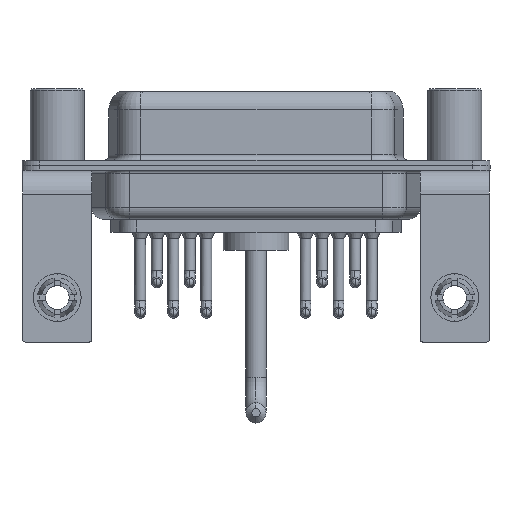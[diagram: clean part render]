
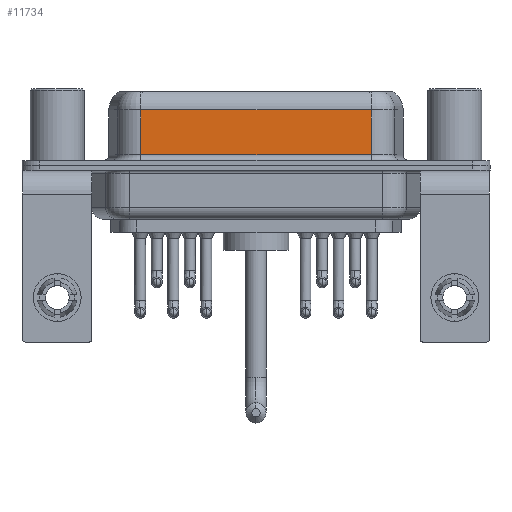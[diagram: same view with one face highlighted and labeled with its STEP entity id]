
A CAD part, front view. The second image highlights one B-rep face of the part: STEP entity #11734.
In plain terms, the highlighted planar face has unit normal (0, -1, 0).
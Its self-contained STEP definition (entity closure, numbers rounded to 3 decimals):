
#398 = DIRECTION ( 'NONE',  ( -1., 0., 0. ) ) ;
#414 = DIRECTION ( 'NONE',  ( 1., 0., 0. ) ) ;
#1727 = LINE ( 'NONE', #19371, #4014 ) ;
#2548 = VERTEX_POINT ( 'NONE', #21222 ) ;
#3657 = CARTESIAN_POINT ( 'NONE',  ( 26.287, -3.95, 6.4 ) ) ;
#3680 = DIRECTION ( 'NONE',  ( 0., 0., -1. ) ) ;
#4014 = VECTOR ( 'NONE', #3680, 1000. ) ;
#4272 = EDGE_CURVE ( 'NONE', #6927, #19515, #12548, .T. ) ;
#4335 = EDGE_CURVE ( 'NONE', #2548, #19515, #21192, .T. ) ;
#4489 = VECTOR ( 'NONE', #398, 1000. ) ;
#5898 = CARTESIAN_POINT ( 'NONE',  ( 7.013, -3.95, 4.65 ) ) ;
#6927 = VERTEX_POINT ( 'NONE', #22051 ) ;
#7411 = EDGE_LOOP ( 'NONE', ( #15290, #13321, #18387, #22272 ) ) ;
#8195 = DIRECTION ( 'NONE',  ( 0., 0., 1. ) ) ;
#8648 = VECTOR ( 'NONE', #414, 1000. ) ;
#9180 = CARTESIAN_POINT ( 'NONE',  ( 26.287, -3.95, 4.65 ) ) ;
#9944 = CARTESIAN_POINT ( 'NONE',  ( 26.287, -3.95, 6.4 ) ) ;
#10717 = DIRECTION ( 'NONE',  ( 0., 0., -1. ) ) ;
#11469 = AXIS2_PLACEMENT_3D ( 'NONE', #9944, #15365, #8195 ) ;
#11734 = ADVANCED_FACE ( 'NONE', ( #15143 ), #13510, .F. ) ;
#12199 = CARTESIAN_POINT ( 'NONE',  ( 26.287, -3.95, 0.9 ) ) ;
#12548 = LINE ( 'NONE', #12199, #8648 ) ;
#12831 = CARTESIAN_POINT ( 'NONE',  ( 26.287, -3.95, 0.9 ) ) ;
#13321 = ORIENTED_EDGE ( 'NONE', *, *, #22125, .T. ) ;
#13510 = PLANE ( 'NONE',  #11469 ) ;
#15143 = FACE_OUTER_BOUND ( 'NONE', #7411, .T. ) ;
#15290 = ORIENTED_EDGE ( 'NONE', *, *, #4335, .F. ) ;
#15365 = DIRECTION ( 'NONE',  ( 0., 1., 0. ) ) ;
#17453 = EDGE_CURVE ( 'NONE', #20867, #6927, #1727, .T. ) ;
#18265 = VECTOR ( 'NONE', #10717, 1000. ) ;
#18387 = ORIENTED_EDGE ( 'NONE', *, *, #17453, .T. ) ;
#19371 = CARTESIAN_POINT ( 'NONE',  ( 7.013, -3.95, 6.4 ) ) ;
#19515 = VERTEX_POINT ( 'NONE', #12831 ) ;
#20867 = VERTEX_POINT ( 'NONE', #5898 ) ;
#21192 = LINE ( 'NONE', #3657, #18265 ) ;
#21222 = CARTESIAN_POINT ( 'NONE',  ( 26.287, -3.95, 4.65 ) ) ;
#21293 = LINE ( 'NONE', #9180, #4489 ) ;
#22051 = CARTESIAN_POINT ( 'NONE',  ( 7.013, -3.95, 0.9 ) ) ;
#22125 = EDGE_CURVE ( 'NONE', #2548, #20867, #21293, .T. ) ;
#22272 = ORIENTED_EDGE ( 'NONE', *, *, #4272, .T. ) ;
